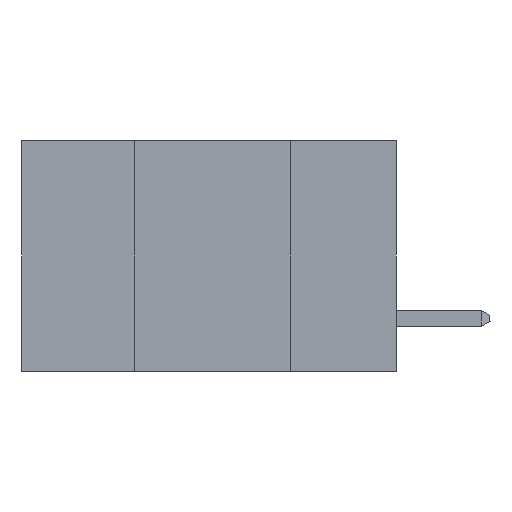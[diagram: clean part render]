
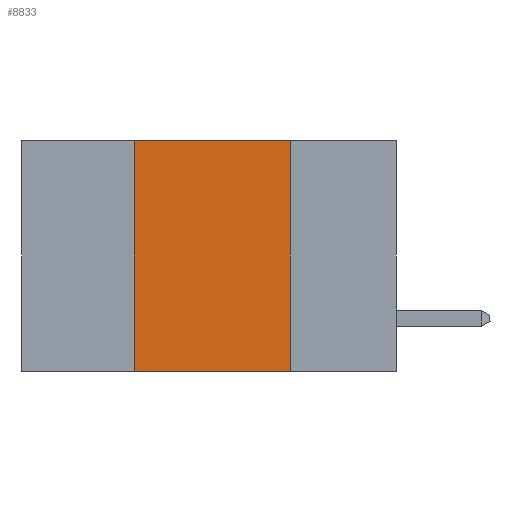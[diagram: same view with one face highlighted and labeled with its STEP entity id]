
A CAD part, left-side view. The second image highlights one B-rep face of the part: STEP entity #8833.
In plain terms, the highlighted planar face has unit normal (-1, 0, 0).
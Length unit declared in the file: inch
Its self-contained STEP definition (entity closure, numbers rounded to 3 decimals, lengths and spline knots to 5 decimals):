
#295 = LINE ( 'NONE', #9836, #5986 ) ;
#1329 = VERTEX_POINT ( 'NONE', #1370 ) ;
#1370 = CARTESIAN_POINT ( 'NONE',  ( 0., 0.42, -0.37 ) ) ;
#3349 = VERTEX_POINT ( 'NONE', #11380 ) ;
#4086 = DIRECTION ( 'NONE',  ( 0., 0., 1. ) ) ;
#4161 = CARTESIAN_POINT ( 'NONE',  ( 0., 0.42, 0. ) ) ;
#4465 = VERTEX_POINT ( 'NONE', #25413 ) ;
#4762 = CARTESIAN_POINT ( 'NONE',  ( 0., 0.6, -0.37 ) ) ;
#5986 = VECTOR ( 'NONE', #19386, 39.37008 ) ;
#8833 = ADVANCED_FACE ( 'NONE', ( #30491 ), #15216, .F. ) ;
#9664 = AXIS2_PLACEMENT_3D ( 'NONE', #15147, #15113, #15039 ) ;
#9836 = CARTESIAN_POINT ( 'NONE',  ( 0., 0.17, 0. ) ) ;
#11380 = CARTESIAN_POINT ( 'NONE',  ( 0., 0.17, 0. ) ) ;
#11972 = EDGE_CURVE ( 'NONE', #1329, #29253, #16679, .T. ) ;
#13188 = VECTOR ( 'NONE', #21791, 39.37008 ) ;
#15039 = DIRECTION ( 'NONE',  ( 0., 0., -1. ) ) ;
#15113 = DIRECTION ( 'NONE',  ( 1., 0., 0. ) ) ;
#15147 = CARTESIAN_POINT ( 'NONE',  ( 0., 0.6, 0. ) ) ;
#15216 = PLANE ( 'NONE',  #9664 ) ;
#16270 = VECTOR ( 'NONE', #16665, 39.37008 ) ;
#16665 = DIRECTION ( 'NONE',  ( 0., -1., 0. ) ) ;
#16679 = LINE ( 'NONE', #4161, #28473 ) ;
#17023 = LINE ( 'NONE', #4762, #16270 ) ;
#17145 = EDGE_LOOP ( 'NONE', ( #22446, #22587, #23207, #23237 ) ) ;
#18013 = LINE ( 'NONE', #19384, #13188 ) ;
#18940 = EDGE_CURVE ( 'NONE', #3349, #4465, #295, .T. ) ;
#19384 = CARTESIAN_POINT ( 'NONE',  ( 0., 0.6, 0. ) ) ;
#19386 = DIRECTION ( 'NONE',  ( 0., 0., -1. ) ) ;
#21533 = CARTESIAN_POINT ( 'NONE',  ( 0., 0.42, 0. ) ) ;
#21733 = EDGE_CURVE ( 'NONE', #1329, #4465, #17023, .T. ) ;
#21791 = DIRECTION ( 'NONE',  ( 0., -1., 0. ) ) ;
#22446 = ORIENTED_EDGE ( 'NONE', *, *, #18940, .F. ) ;
#22587 = ORIENTED_EDGE ( 'NONE', *, *, #27661, .F. ) ;
#23207 = ORIENTED_EDGE ( 'NONE', *, *, #11972, .F. ) ;
#23237 = ORIENTED_EDGE ( 'NONE', *, *, #21733, .T. ) ;
#25413 = CARTESIAN_POINT ( 'NONE',  ( 0., 0.17, -0.37 ) ) ;
#27661 = EDGE_CURVE ( 'NONE', #29253, #3349, #18013, .T. ) ;
#28473 = VECTOR ( 'NONE', #4086, 39.37008 ) ;
#29253 = VERTEX_POINT ( 'NONE', #21533 ) ;
#30491 = FACE_OUTER_BOUND ( 'NONE', #17145, .T. ) ;
